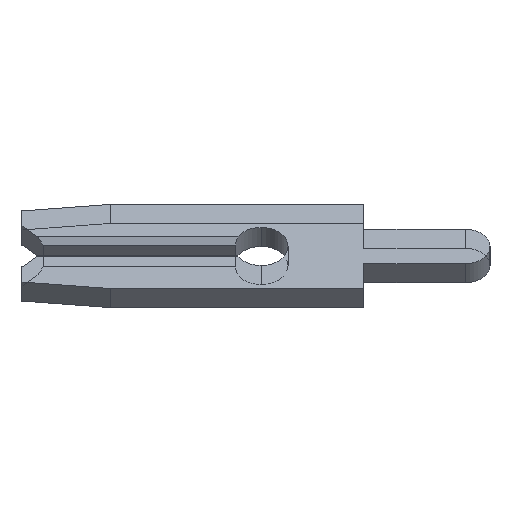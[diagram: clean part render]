
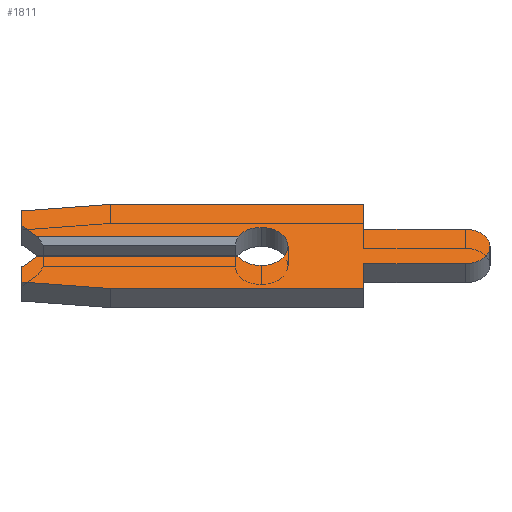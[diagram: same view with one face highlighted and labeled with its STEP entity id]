
A CAD part, left-side view. The second image highlights one B-rep face of the part: STEP entity #1811.
In plain terms, the highlighted face is planar.
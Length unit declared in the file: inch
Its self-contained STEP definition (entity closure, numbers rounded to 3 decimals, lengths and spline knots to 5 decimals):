
#3 = ORIENTED_EDGE ( 'NONE', *, *, #1937, .F. ) ;
#4 = VERTEX_POINT ( 'NONE', #409 ) ;
#16 = VECTOR ( 'NONE', #1229, 39.37008 ) ;
#67 = CARTESIAN_POINT ( 'NONE',  ( -0.013, 0.231, 0.013 ) ) ;
#69 = ORIENTED_EDGE ( 'NONE', *, *, #2318, .F. ) ;
#80 = CARTESIAN_POINT ( 'NONE',  ( -0.013, -0.099, 0.0575 ) ) ;
#97 = ORIENTED_EDGE ( 'NONE', *, *, #1604, .F. ) ;
#109 = VECTOR ( 'NONE', #456, 39.37008 ) ;
#111 = VECTOR ( 'NONE', #1974, 39.37008 ) ;
#158 = CARTESIAN_POINT ( 'NONE',  ( -0.013, 0.146, -0.0575 ) ) ;
#176 = DIRECTION ( 'NONE',  ( 0., 1., 0. ) ) ;
#181 = EDGE_CURVE ( 'NONE', #1450, #1830, #1557, .T. ) ;
#189 = VERTEX_POINT ( 'NONE', #2163 ) ;
#217 = EDGE_CURVE ( 'NONE', #1830, #2046, #426, .T. ) ;
#237 = DIRECTION ( 'NONE',  ( 0., -0.707, 0.707 ) ) ;
#242 = CARTESIAN_POINT ( 'NONE',  ( -0.013, 0.231, -0.028 ) ) ;
#294 = CARTESIAN_POINT ( 'NONE',  ( -0.013, -0.099, -0.0575 ) ) ;
#300 = CARTESIAN_POINT ( 'NONE',  ( -0.013, 0., 0. ) ) ;
#350 = EDGE_CURVE ( 'NONE', #2387, #1450, #1826, .T. ) ;
#390 = AXIS2_PLACEMENT_3D ( 'NONE', #300, #681, #2373 ) ;
#402 = EDGE_CURVE ( 'NONE', #189, #1242, #1584, .T. ) ;
#406 = VERTEX_POINT ( 'NONE', #1587 ) ;
#409 = CARTESIAN_POINT ( 'NONE',  ( -0.013, -0.1975, -0.0235 ) ) ;
#426 = LINE ( 'NONE', #2336, #111 ) ;
#434 = CARTESIAN_POINT ( 'NONE',  ( -0.013, 0.2105, -0.0075 ) ) ;
#435 = EDGE_CURVE ( 'NONE', #1151, #1954, #2331, .T. ) ;
#440 = ORIENTED_EDGE ( 'NONE', *, *, #560, .F. ) ;
#456 = DIRECTION ( 'NONE',  ( 0., -1., 0. ) ) ;
#505 = PLANE ( 'NONE',  #1023 ) ;
#511 = CARTESIAN_POINT ( 'NONE',  ( -0.013, 0., 0.026 ) ) ;
#560 = EDGE_CURVE ( 'NONE', #886, #1242, #2149, .T. ) ;
#567 = VECTOR ( 'NONE', #176, 39.37008 ) ;
#601 = VECTOR ( 'NONE', #1095, 39.37008 ) ;
#615 = ORIENTED_EDGE ( 'NONE', *, *, #995, .F. ) ;
#618 = DIRECTION ( 'NONE',  ( 0., 0., 1. ) ) ;
#631 = CIRCLE ( 'NONE', #2014, 0.0235 ) ;
#647 = ORIENTED_EDGE ( 'NONE', *, *, #1911, .F. ) ;
#656 = VECTOR ( 'NONE', #863, 39.37008 ) ;
#659 = AXIS2_PLACEMENT_3D ( 'NONE', #677, #2189, #1641 ) ;
#677 = CARTESIAN_POINT ( 'NONE',  ( -0.013, 0., 0. ) ) ;
#681 = DIRECTION ( 'NONE',  ( -1., 0., 0. ) ) ;
#697 = VECTOR ( 'NONE', #237, 39.37008 ) ;
#702 = CARTESIAN_POINT ( 'NONE',  ( -0.013, 0.231, 0.04857 ) ) ;
#711 = VERTEX_POINT ( 'NONE', #1254 ) ;
#725 = CARTESIAN_POINT ( 'NONE',  ( -0.013, -0.099, 0.0235 ) ) ;
#728 = VERTEX_POINT ( 'NONE', #1234 ) ;
#730 = DIRECTION ( 'NONE',  ( 0., 0.707, 0.707 ) ) ;
#734 = DIRECTION ( 'NONE',  ( 0., 0.995, 0.105 ) ) ;
#847 = EDGE_CURVE ( 'NONE', #2071, #406, #1317, .T. ) ;
#857 = DIRECTION ( 'NONE',  ( 0., 0., -1. ) ) ;
#863 = DIRECTION ( 'NONE',  ( 0., -0.995, 0.105 ) ) ;
#869 = EDGE_CURVE ( 'NONE', #2067, #1522, #1135, .T. ) ;
#877 = CARTESIAN_POINT ( 'NONE',  ( -0.013, 0.231, 0.028 ) ) ;
#886 = VERTEX_POINT ( 'NONE', #511 ) ;
#907 = CARTESIAN_POINT ( 'NONE',  ( -0.013, -0.1975, 0. ) ) ;
#911 = CARTESIAN_POINT ( 'NONE',  ( -0.013, 0.231, -0.04857 ) ) ;
#918 = LINE ( 'NONE', #158, #567 ) ;
#941 = ORIENTED_EDGE ( 'NONE', *, *, #869, .F. ) ;
#942 = VERTEX_POINT ( 'NONE', #2234 ) ;
#995 = EDGE_CURVE ( 'NONE', #189, #1151, #1941, .T. ) ;
#1003 = ORIENTED_EDGE ( 'NONE', *, *, #2112, .F. ) ;
#1020 = VECTOR ( 'NONE', #618, 39.37008 ) ;
#1023 = AXIS2_PLACEMENT_3D ( 'NONE', #2010, #2219, #857 ) ;
#1044 = CARTESIAN_POINT ( 'NONE',  ( -0.013, -0.099, 0.0235 ) ) ;
#1050 = CARTESIAN_POINT ( 'NONE',  ( -0.013, 0.02252, -0.013 ) ) ;
#1059 = CARTESIAN_POINT ( 'NONE',  ( -0.013, 0.146, 0.0575 ) ) ;
#1095 = DIRECTION ( 'NONE',  ( 0., -1., 0. ) ) ;
#1135 = LINE ( 'NONE', #2426, #2001 ) ;
#1151 = VERTEX_POINT ( 'NONE', #2051 ) ;
#1160 = VECTOR ( 'NONE', #1834, 39.37008 ) ;
#1166 = VECTOR ( 'NONE', #1701, 39.37008 ) ;
#1185 = ORIENTED_EDGE ( 'NONE', *, *, #435, .F. ) ;
#1215 = EDGE_CURVE ( 'NONE', #406, #4, #631, .T. ) ;
#1223 = CIRCLE ( 'NONE', #2093, 0.026 ) ;
#1224 = ORIENTED_EDGE ( 'NONE', *, *, #217, .F. ) ;
#1229 = DIRECTION ( 'NONE',  ( 0., 0., -1. ) ) ;
#1234 = CARTESIAN_POINT ( 'NONE',  ( -0.013, 0., -0.026 ) ) ;
#1242 = VERTEX_POINT ( 'NONE', #1905 ) ;
#1254 = CARTESIAN_POINT ( 'NONE',  ( -0.013, -0.099, -0.0235 ) ) ;
#1263 = DIRECTION ( 'NONE',  ( 0., 0., -1. ) ) ;
#1317 = LINE ( 'NONE', #725, #601 ) ;
#1332 = VERTEX_POINT ( 'NONE', #1341 ) ;
#1341 = CARTESIAN_POINT ( 'NONE',  ( -0.013, -0.099, -0.0575 ) ) ;
#1397 = LINE ( 'NONE', #2018, #656 ) ;
#1450 = VERTEX_POINT ( 'NONE', #2295 ) ;
#1458 = CIRCLE ( 'NONE', #390, 0.026 ) ;
#1465 = EDGE_CURVE ( 'NONE', #4, #711, #1672, .T. ) ;
#1468 = CARTESIAN_POINT ( 'NONE',  ( -0.013, 0.2105, 0.0075 ) ) ;
#1496 = DIRECTION ( 'NONE',  ( 0., 0., 1. ) ) ;
#1521 = DIRECTION ( 'NONE',  ( 1., 0., 0. ) ) ;
#1522 = VERTEX_POINT ( 'NONE', #1689 ) ;
#1557 = LINE ( 'NONE', #434, #697 ) ;
#1570 = ORIENTED_EDGE ( 'NONE', *, *, #847, .F. ) ;
#1582 = LINE ( 'NONE', #80, #16 ) ;
#1584 = LINE ( 'NONE', #67, #109 ) ;
#1587 = CARTESIAN_POINT ( 'NONE',  ( -0.013, -0.1975, 0.0235 ) ) ;
#1601 = ORIENTED_EDGE ( 'NONE', *, *, #1766, .F. ) ;
#1604 = EDGE_CURVE ( 'NONE', #1332, #942, #918, .T. ) ;
#1626 = CARTESIAN_POINT ( 'NONE',  ( -0.013, 0., 0. ) ) ;
#1634 = CARTESIAN_POINT ( 'NONE',  ( -0.013, 0.216, -0.013 ) ) ;
#1641 = DIRECTION ( 'NONE',  ( 0., 0., -1. ) ) ;
#1660 = ORIENTED_EDGE ( 'NONE', *, *, #402, .T. ) ;
#1672 = LINE ( 'NONE', #2279, #1166 ) ;
#1689 = CARTESIAN_POINT ( 'NONE',  ( -0.013, -0.099, 0.0575 ) ) ;
#1701 = DIRECTION ( 'NONE',  ( 0., 1., 0. ) ) ;
#1766 = EDGE_CURVE ( 'NONE', #2046, #728, #1458, .T. ) ;
#1779 = ORIENTED_EDGE ( 'NONE', *, *, #350, .F. ) ;
#1811 = ADVANCED_FACE ( 'NONE', ( #1873 ), #505, .F. ) ;
#1820 = DIRECTION ( 'NONE',  ( -1., 0., 0. ) ) ;
#1821 = VECTOR ( 'NONE', #730, 39.37008 ) ;
#1826 = LINE ( 'NONE', #242, #1020 ) ;
#1830 = VERTEX_POINT ( 'NONE', #1634 ) ;
#1834 = DIRECTION ( 'NONE',  ( 0., 0., -1. ) ) ;
#1839 = DIRECTION ( 'NONE',  ( 0., -1., 0. ) ) ;
#1873 = FACE_OUTER_BOUND ( 'NONE', #2231, .T. ) ;
#1905 = CARTESIAN_POINT ( 'NONE',  ( -0.013, 0.02252, 0.013 ) ) ;
#1908 = VECTOR ( 'NONE', #734, 39.37008 ) ;
#1911 = EDGE_CURVE ( 'NONE', #711, #1332, #2443, .T. ) ;
#1913 = ORIENTED_EDGE ( 'NONE', *, *, #181, .F. ) ;
#1937 = EDGE_CURVE ( 'NONE', #1954, #2067, #1397, .T. ) ;
#1941 = LINE ( 'NONE', #1468, #1821 ) ;
#1954 = VERTEX_POINT ( 'NONE', #702 ) ;
#1972 = ORIENTED_EDGE ( 'NONE', *, *, #2058, .F. ) ;
#1974 = DIRECTION ( 'NONE',  ( 0., -1., 0. ) ) ;
#2001 = VECTOR ( 'NONE', #1839, 39.37008 ) ;
#2010 = CARTESIAN_POINT ( 'NONE',  ( -0.013, 0., 0. ) ) ;
#2014 = AXIS2_PLACEMENT_3D ( 'NONE', #907, #1521, #1496 ) ;
#2018 = CARTESIAN_POINT ( 'NONE',  ( -0.013, 0.231, 0.04857 ) ) ;
#2046 = VERTEX_POINT ( 'NONE', #1050 ) ;
#2051 = CARTESIAN_POINT ( 'NONE',  ( -0.013, 0.231, 0.028 ) ) ;
#2058 = EDGE_CURVE ( 'NONE', #1522, #2071, #1582, .T. ) ;
#2067 = VERTEX_POINT ( 'NONE', #1059 ) ;
#2071 = VERTEX_POINT ( 'NONE', #1044 ) ;
#2085 = VECTOR ( 'NONE', #2198, 39.37008 ) ;
#2093 = AXIS2_PLACEMENT_3D ( 'NONE', #1626, #1820, #1263 ) ;
#2107 = ORIENTED_EDGE ( 'NONE', *, *, #1215, .F. ) ;
#2109 = ORIENTED_EDGE ( 'NONE', *, *, #1465, .F. ) ;
#2112 = EDGE_CURVE ( 'NONE', #728, #886, #1223, .T. ) ;
#2149 = CIRCLE ( 'NONE', #659, 0.026 ) ;
#2163 = CARTESIAN_POINT ( 'NONE',  ( -0.013, 0.216, 0.013 ) ) ;
#2189 = DIRECTION ( 'NONE',  ( -1., 0., 0. ) ) ;
#2198 = DIRECTION ( 'NONE',  ( 0., 0., 1. ) ) ;
#2219 = DIRECTION ( 'NONE',  ( 1., 0., 0. ) ) ;
#2228 = CARTESIAN_POINT ( 'NONE',  ( -0.013, 0.231, -0.04857 ) ) ;
#2231 = EDGE_LOOP ( 'NONE', ( #1660, #440, #1003, #1601, #1224, #1913, #1779, #69, #97, #647, #2109, #2107, #1570, #1972, #941, #3, #1185, #615 ) ) ;
#2234 = CARTESIAN_POINT ( 'NONE',  ( -0.013, 0.146, -0.0575 ) ) ;
#2279 = CARTESIAN_POINT ( 'NONE',  ( -0.013, -0.099, -0.0235 ) ) ;
#2295 = CARTESIAN_POINT ( 'NONE',  ( -0.013, 0.231, -0.028 ) ) ;
#2318 = EDGE_CURVE ( 'NONE', #942, #2387, #2420, .T. ) ;
#2331 = LINE ( 'NONE', #877, #2085 ) ;
#2336 = CARTESIAN_POINT ( 'NONE',  ( -0.013, 0., -0.013 ) ) ;
#2373 = DIRECTION ( 'NONE',  ( 0., 0., -1. ) ) ;
#2387 = VERTEX_POINT ( 'NONE', #911 ) ;
#2420 = LINE ( 'NONE', #2228, #1908 ) ;
#2426 = CARTESIAN_POINT ( 'NONE',  ( -0.013, 0.146, 0.0575 ) ) ;
#2443 = LINE ( 'NONE', #294, #1160 ) ;
